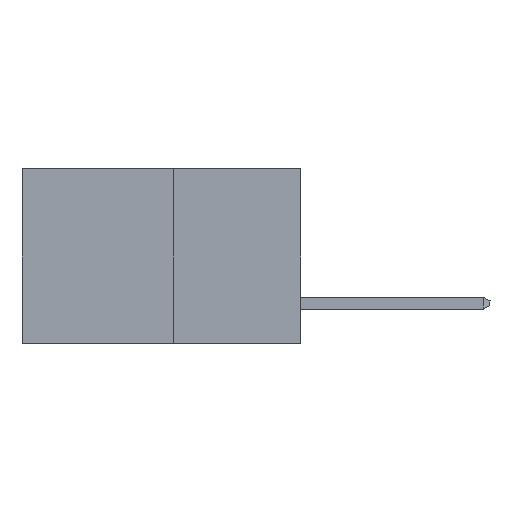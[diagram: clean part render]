
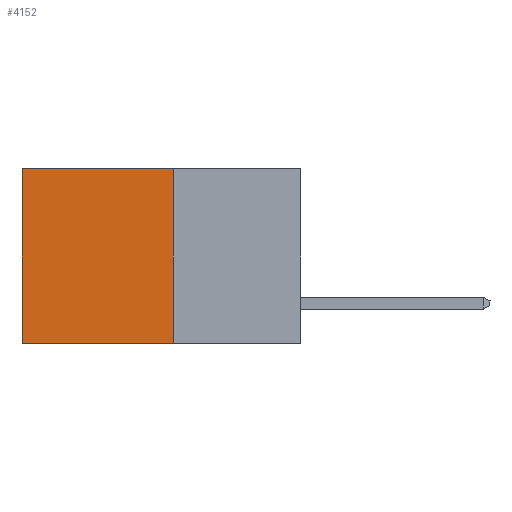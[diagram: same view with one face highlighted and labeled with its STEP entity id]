
A CAD part, left-side view. The second image highlights one B-rep face of the part: STEP entity #4152.
In plain terms, the highlighted planar face has unit normal (-1, 0, 0).
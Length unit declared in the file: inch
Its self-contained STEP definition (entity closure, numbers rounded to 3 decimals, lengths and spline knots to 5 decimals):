
#857 = ORIENTED_EDGE ( 'NONE', *, *, #22983, .T. ) ;
#1056 = AXIS2_PLACEMENT_3D ( 'NONE', #24537, #27000, #25031 ) ;
#1893 = DIRECTION ( 'NONE',  ( 0., 1., 0. ) ) ;
#1895 = EDGE_LOOP ( 'NONE', ( #857, #27783, #10698, #6792 ) ) ;
#2223 = CARTESIAN_POINT ( 'NONE',  ( 0.277, 0.27, -0.37 ) ) ;
#2713 = LINE ( 'NONE', #9732, #28536 ) ;
#4152 = ADVANCED_FACE ( 'NONE', ( #7973 ), #23037, .F. ) ;
#4676 = VECTOR ( 'NONE', #6594, 39.37008 ) ;
#5289 = VERTEX_POINT ( 'NONE', #5453 ) ;
#5453 = CARTESIAN_POINT ( 'NONE',  ( 0.277, 0.27, 0. ) ) ;
#6594 = DIRECTION ( 'NONE',  ( 0., 0., -1. ) ) ;
#6792 = ORIENTED_EDGE ( 'NONE', *, *, #21130, .T. ) ;
#7515 = VERTEX_POINT ( 'NONE', #7532 ) ;
#7532 = CARTESIAN_POINT ( 'NONE',  ( 0.277, 0.59, -0.37 ) ) ;
#7973 = FACE_OUTER_BOUND ( 'NONE', #1895, .T. ) ;
#8499 = VERTEX_POINT ( 'NONE', #26236 ) ;
#9732 = CARTESIAN_POINT ( 'NONE',  ( 0.277, 0.27, -0.37 ) ) ;
#10698 = ORIENTED_EDGE ( 'NONE', *, *, #31212, .F. ) ;
#11242 = VECTOR ( 'NONE', #22512, 39.37008 ) ;
#11899 = CARTESIAN_POINT ( 'NONE',  ( 0.277, 0.59, -0.37 ) ) ;
#14300 = LINE ( 'NONE', #2223, #20239 ) ;
#19883 = CARTESIAN_POINT ( 'NONE',  ( 0.277, 0.27, 0. ) ) ;
#20239 = VECTOR ( 'NONE', #25489, 39.37008 ) ;
#21130 = EDGE_CURVE ( 'NONE', #5289, #28127, #24895, .T. ) ;
#22419 = EDGE_CURVE ( 'NONE', #8499, #7515, #2713, .T. ) ;
#22512 = DIRECTION ( 'NONE',  ( 0., 1., 0. ) ) ;
#22983 = EDGE_CURVE ( 'NONE', #28127, #7515, #31288, .T. ) ;
#23037 = PLANE ( 'NONE',  #1056 ) ;
#24537 = CARTESIAN_POINT ( 'NONE',  ( 0.277, 0.27, -0.37 ) ) ;
#24895 = LINE ( 'NONE', #19883, #11242 ) ;
#25031 = DIRECTION ( 'NONE',  ( 0., 0., -1. ) ) ;
#25433 = CARTESIAN_POINT ( 'NONE',  ( 0.277, 0.59, 0. ) ) ;
#25489 = DIRECTION ( 'NONE',  ( 0., 0., -1. ) ) ;
#26236 = CARTESIAN_POINT ( 'NONE',  ( 0.277, 0.27, -0.37 ) ) ;
#27000 = DIRECTION ( 'NONE',  ( 1., 0., 0. ) ) ;
#27783 = ORIENTED_EDGE ( 'NONE', *, *, #22419, .F. ) ;
#28127 = VERTEX_POINT ( 'NONE', #25433 ) ;
#28536 = VECTOR ( 'NONE', #1893, 39.37008 ) ;
#31212 = EDGE_CURVE ( 'NONE', #5289, #8499, #14300, .T. ) ;
#31288 = LINE ( 'NONE', #11899, #4676 ) ;
